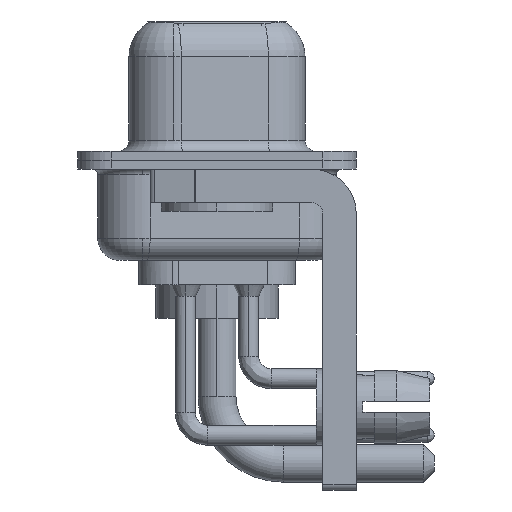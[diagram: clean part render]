
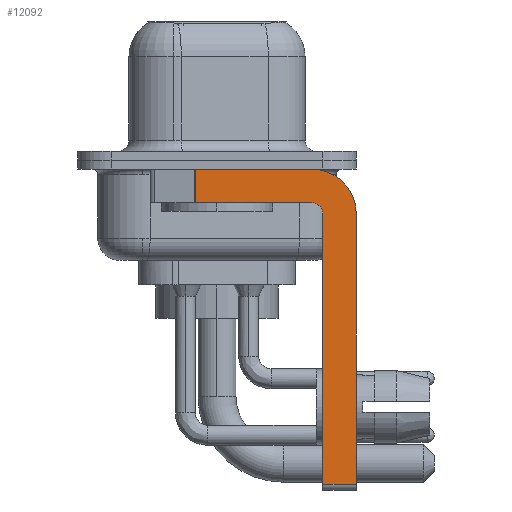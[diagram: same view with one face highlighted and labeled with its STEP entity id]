
A CAD part, left-side view. The second image highlights one B-rep face of the part: STEP entity #12092.
In plain terms, the highlighted planar face has unit normal (-1, 0, 0).
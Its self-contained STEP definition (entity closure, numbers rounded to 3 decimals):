
#1 = EDGE_CURVE ( 'NONE', #1929, #8538, #17022, .T. ) ;
#528 = DIRECTION ( 'NONE',  ( 0., -1., 0. ) ) ;
#771 = DIRECTION ( 'NONE',  ( 1., 0., 0. ) ) ;
#1929 = VERTEX_POINT ( 'NONE', #5865 ) ;
#2028 = EDGE_CURVE ( 'NONE', #3749, #11755, #14475, .T. ) ;
#2212 = DIRECTION ( 'NONE',  ( 0., 0., 1. ) ) ;
#3128 = CIRCLE ( 'NONE', #11295, 2. ) ;
#3249 = ORIENTED_EDGE ( 'NONE', *, *, #4292, .F. ) ;
#3594 = CARTESIAN_POINT ( 'NONE',  ( -2.9, -4.25, -2.4 ) ) ;
#3749 = VERTEX_POINT ( 'NONE', #16938 ) ;
#4003 = CARTESIAN_POINT ( 'NONE',  ( -2.9, -4.25, -2.4 ) ) ;
#4238 = ORIENTED_EDGE ( 'NONE', *, *, #1, .F. ) ;
#4292 = EDGE_CURVE ( 'NONE', #3749, #8935, #13277, .T. ) ;
#4848 = CARTESIAN_POINT ( 'NONE',  ( -2.9, -4.75, -2.4 ) ) ;
#5138 = EDGE_CURVE ( 'NONE', #8935, #1929, #3128, .T. ) ;
#5513 = DIRECTION ( 'NONE',  ( 0., 0., -1. ) ) ;
#5686 = CARTESIAN_POINT ( 'NONE',  ( -2.9, -4.25, -14.55 ) ) ;
#5865 = CARTESIAN_POINT ( 'NONE',  ( -2.9, -6.25, -2.4 ) ) ;
#6511 = EDGE_LOOP ( 'NONE', ( #3249, #11239, #17493, #10708, #7563, #8095, #4238, #18385 ) ) ;
#7133 = DIRECTION ( 'NONE',  ( 1., 0., 0. ) ) ;
#7563 = ORIENTED_EDGE ( 'NONE', *, *, #14034, .F. ) ;
#7698 = VECTOR ( 'NONE', #12781, 1000. ) ;
#7704 = CARTESIAN_POINT ( 'NONE',  ( -2.9, -4.25, -2.4 ) ) ;
#8095 = ORIENTED_EDGE ( 'NONE', *, *, #16451, .T. ) ;
#8348 = CARTESIAN_POINT ( 'NONE',  ( -2.9, -6.25, -2.4 ) ) ;
#8451 = CARTESIAN_POINT ( 'NONE',  ( -2.9, -4.25, -1.9 ) ) ;
#8538 = VERTEX_POINT ( 'NONE', #9241 ) ;
#8644 = PLANE ( 'NONE',  #17186 ) ;
#8689 = VECTOR ( 'NONE', #12952, 1000. ) ;
#8897 = DIRECTION ( 'NONE',  ( 0., -1., 0. ) ) ;
#8935 = VERTEX_POINT ( 'NONE', #14546 ) ;
#9241 = CARTESIAN_POINT ( 'NONE',  ( -2.9, -6.25, -14.55 ) ) ;
#10046 = LINE ( 'NONE', #5686, #13991 ) ;
#10051 = CARTESIAN_POINT ( 'NONE',  ( -2.9, 0.978, -1.9 ) ) ;
#10708 = ORIENTED_EDGE ( 'NONE', *, *, #16096, .F. ) ;
#10778 = VECTOR ( 'NONE', #528, 1000. ) ;
#10882 = CARTESIAN_POINT ( 'NONE',  ( -2.9, -4.25, -1.9 ) ) ;
#11239 = ORIENTED_EDGE ( 'NONE', *, *, #2028, .T. ) ;
#11295 = AXIS2_PLACEMENT_3D ( 'NONE', #3594, #771, #18066 ) ;
#11755 = VERTEX_POINT ( 'NONE', #11862 ) ;
#11862 = CARTESIAN_POINT ( 'NONE',  ( -2.9, 0.978, -1.9 ) ) ;
#12092 = ADVANCED_FACE ( 'NONE', ( #15475 ), #8644, .F. ) ;
#12170 = VECTOR ( 'NONE', #16442, 1000. ) ;
#12781 = DIRECTION ( 'NONE',  ( 0., 1., 0. ) ) ;
#12952 = DIRECTION ( 'NONE',  ( 0., 0., -1. ) ) ;
#13185 = CARTESIAN_POINT ( 'NONE',  ( -2.9, 3., -0.4 ) ) ;
#13277 = LINE ( 'NONE', #13185, #10778 ) ;
#13335 = VERTEX_POINT ( 'NONE', #10882 ) ;
#13967 = AXIS2_PLACEMENT_3D ( 'NONE', #7704, #15269, #2212 ) ;
#13991 = VECTOR ( 'NONE', #8897, 1000. ) ;
#14034 = EDGE_CURVE ( 'NONE', #17421, #16177, #14401, .T. ) ;
#14251 = CIRCLE ( 'NONE', #13967, 0.5 ) ;
#14401 = LINE ( 'NONE', #16961, #14803 ) ;
#14475 = LINE ( 'NONE', #10051, #12170 ) ;
#14546 = CARTESIAN_POINT ( 'NONE',  ( -2.9, -4.25, -0.4 ) ) ;
#14803 = VECTOR ( 'NONE', #18549, 1000. ) ;
#15269 = DIRECTION ( 'NONE',  ( -1., 0., 0. ) ) ;
#15475 = FACE_OUTER_BOUND ( 'NONE', #6511, .T. ) ;
#16096 = EDGE_CURVE ( 'NONE', #16177, #13335, #14251, .T. ) ;
#16177 = VERTEX_POINT ( 'NONE', #4848 ) ;
#16304 = CARTESIAN_POINT ( 'NONE',  ( -2.9, -4.75, -14.55 ) ) ;
#16442 = DIRECTION ( 'NONE',  ( 0., 0., -1. ) ) ;
#16451 = EDGE_CURVE ( 'NONE', #17421, #8538, #10046, .T. ) ;
#16938 = CARTESIAN_POINT ( 'NONE',  ( -2.9, 0.978, -0.4 ) ) ;
#16961 = CARTESIAN_POINT ( 'NONE',  ( -2.9, -4.75, -14.8 ) ) ;
#17022 = LINE ( 'NONE', #8348, #8689 ) ;
#17186 = AXIS2_PLACEMENT_3D ( 'NONE', #4003, #7133, #5513 ) ;
#17421 = VERTEX_POINT ( 'NONE', #16304 ) ;
#17493 = ORIENTED_EDGE ( 'NONE', *, *, #17581, .F. ) ;
#17581 = EDGE_CURVE ( 'NONE', #13335, #11755, #18456, .T. ) ;
#18066 = DIRECTION ( 'NONE',  ( 0., 0., -1. ) ) ;
#18385 = ORIENTED_EDGE ( 'NONE', *, *, #5138, .F. ) ;
#18456 = LINE ( 'NONE', #8451, #7698 ) ;
#18549 = DIRECTION ( 'NONE',  ( 0., 0., 1. ) ) ;
